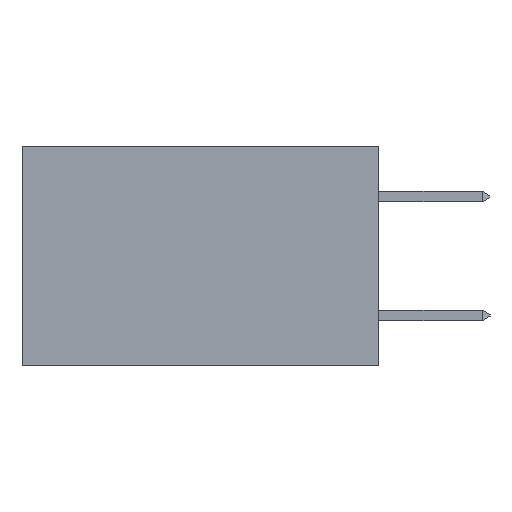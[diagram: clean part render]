
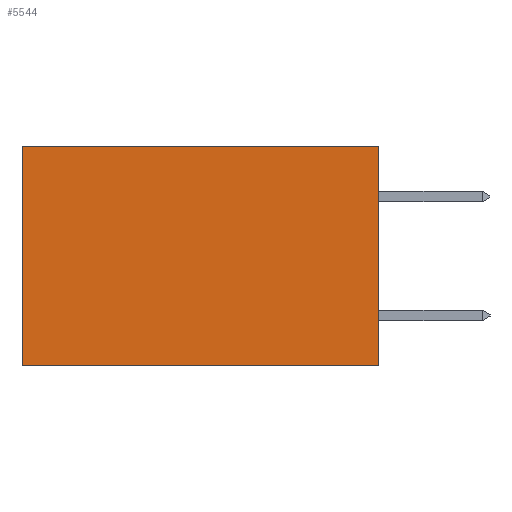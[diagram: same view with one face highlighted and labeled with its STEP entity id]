
A CAD part, left-side view. The second image highlights one B-rep face of the part: STEP entity #5544.
In plain terms, the highlighted planar face has unit normal (-1, 0, 0).
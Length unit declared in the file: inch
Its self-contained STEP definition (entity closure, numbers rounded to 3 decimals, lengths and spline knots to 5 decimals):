
#497 = EDGE_CURVE ( 'NONE', #6347, #7734, #7510, .T. ) ;
#569 = EDGE_CURVE ( 'NONE', #2090, #6347, #5988, .T. ) ;
#638 = CARTESIAN_POINT ( 'NONE',  ( 0.2615, 0., -0.37 ) ) ;
#2090 = VERTEX_POINT ( 'NONE', #10441 ) ;
#2460 = EDGE_LOOP ( 'NONE', ( #11702, #2611, #7404, #12061 ) ) ;
#2611 = ORIENTED_EDGE ( 'NONE', *, *, #497, .F. ) ;
#3133 = VECTOR ( 'NONE', #4220, 39.37008 ) ;
#3896 = EDGE_CURVE ( 'NONE', #2090, #6339, #5647, .T. ) ;
#4174 = DIRECTION ( 'NONE',  ( 0., 0., -1. ) ) ;
#4220 = DIRECTION ( 'NONE',  ( 0., 0., -1. ) ) ;
#4265 = CARTESIAN_POINT ( 'NONE',  ( 0.2615, 0.6, -0.37 ) ) ;
#4266 = DIRECTION ( 'NONE',  ( 0., 1., 0. ) ) ;
#4285 = CARTESIAN_POINT ( 'NONE',  ( 0.2615, 0., 0. ) ) ;
#4851 = VECTOR ( 'NONE', #6547, 39.37008 ) ;
#5000 = EDGE_CURVE ( 'NONE', #6339, #7734, #6201, .T. ) ;
#5544 = ADVANCED_FACE ( 'NONE', ( #10382 ), #12244, .F. ) ;
#5567 = DIRECTION ( 'NONE',  ( 0., 0., -1. ) ) ;
#5647 = LINE ( 'NONE', #4285, #10426 ) ;
#5988 = LINE ( 'NONE', #638, #3133 ) ;
#6152 = CARTESIAN_POINT ( 'NONE',  ( 0.2615, 0., -0.37 ) ) ;
#6201 = LINE ( 'NONE', #4265, #8433 ) ;
#6339 = VERTEX_POINT ( 'NONE', #8373 ) ;
#6347 = VERTEX_POINT ( 'NONE', #8829 ) ;
#6547 = DIRECTION ( 'NONE',  ( 0., 1., 0. ) ) ;
#7404 = ORIENTED_EDGE ( 'NONE', *, *, #569, .F. ) ;
#7510 = LINE ( 'NONE', #6152, #4851 ) ;
#7734 = VERTEX_POINT ( 'NONE', #9486 ) ;
#8373 = CARTESIAN_POINT ( 'NONE',  ( 0.2615, 0.6, 0. ) ) ;
#8433 = VECTOR ( 'NONE', #4174, 39.37008 ) ;
#8829 = CARTESIAN_POINT ( 'NONE',  ( 0.2615, 0., -0.37 ) ) ;
#9486 = CARTESIAN_POINT ( 'NONE',  ( 0.2615, 0.6, -0.37 ) ) ;
#10382 = FACE_OUTER_BOUND ( 'NONE', #2460, .T. ) ;
#10426 = VECTOR ( 'NONE', #4266, 39.37008 ) ;
#10441 = CARTESIAN_POINT ( 'NONE',  ( 0.2615, 0., 0. ) ) ;
#11702 = ORIENTED_EDGE ( 'NONE', *, *, #5000, .T. ) ;
#11801 = DIRECTION ( 'NONE',  ( 1., 0., 0. ) ) ;
#11984 = AXIS2_PLACEMENT_3D ( 'NONE', #12143, #11801, #5567 ) ;
#12061 = ORIENTED_EDGE ( 'NONE', *, *, #3896, .T. ) ;
#12143 = CARTESIAN_POINT ( 'NONE',  ( 0.2615, 0., -0.37 ) ) ;
#12244 = PLANE ( 'NONE',  #11984 ) ;
